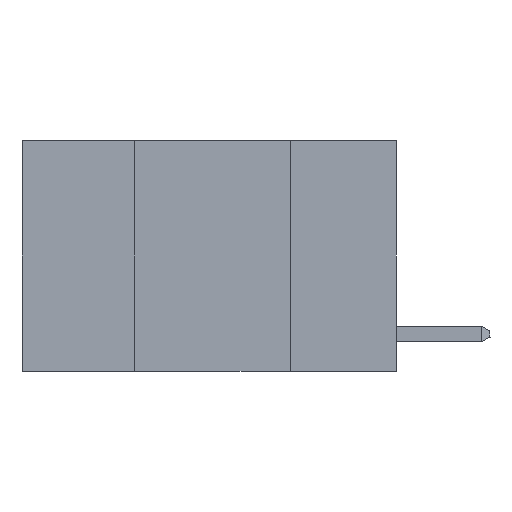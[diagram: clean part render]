
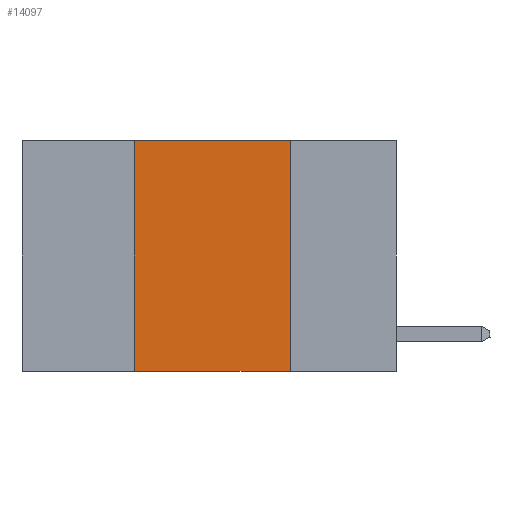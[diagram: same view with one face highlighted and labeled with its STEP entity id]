
A CAD part, left-side view. The second image highlights one B-rep face of the part: STEP entity #14097.
In plain terms, the highlighted planar face has unit normal (-1, 0, 0).
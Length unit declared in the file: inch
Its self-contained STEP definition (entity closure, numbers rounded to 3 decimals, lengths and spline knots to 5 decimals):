
#681 = FACE_OUTER_BOUND ( 'NONE', #6079, .T. ) ;
#1766 = DIRECTION ( 'NONE',  ( 0., -1., 0. ) ) ;
#2060 = ORIENTED_EDGE ( 'NONE', *, *, #2800, .F. ) ;
#2800 = EDGE_CURVE ( 'NONE', #11734, #18228, #6133, .T. ) ;
#3942 = DIRECTION ( 'NONE',  ( 0., 0., -1. ) ) ;
#5501 = DIRECTION ( 'NONE',  ( 0., 0., 1. ) ) ;
#6079 = EDGE_LOOP ( 'NONE', ( #2060, #16665, #7843, #17218 ) ) ;
#6133 = LINE ( 'NONE', #7042, #19045 ) ;
#6497 = LINE ( 'NONE', #8415, #15768 ) ;
#6678 = EDGE_CURVE ( 'NONE', #20570, #18228, #6497, .T. ) ;
#7042 = CARTESIAN_POINT ( 'NONE',  ( 0., 0.17, 0. ) ) ;
#7843 = ORIENTED_EDGE ( 'NONE', *, *, #19462, .F. ) ;
#8415 = CARTESIAN_POINT ( 'NONE',  ( 0., 0.6, -0.37 ) ) ;
#8796 = VECTOR ( 'NONE', #1766, 39.37008 ) ;
#11658 = EDGE_CURVE ( 'NONE', #17234, #11734, #13452, .T. ) ;
#11734 = VERTEX_POINT ( 'NONE', #17817 ) ;
#11872 = DIRECTION ( 'NONE',  ( 0., -1., 0. ) ) ;
#12657 = CARTESIAN_POINT ( 'NONE',  ( 0., 0.6, 0. ) ) ;
#13268 = CARTESIAN_POINT ( 'NONE',  ( 0., 0.42, 0. ) ) ;
#13452 = LINE ( 'NONE', #15804, #8796 ) ;
#14097 = ADVANCED_FACE ( 'NONE', ( #681 ), #19725, .F. ) ;
#14164 = CARTESIAN_POINT ( 'NONE',  ( 0., 0.42, 0. ) ) ;
#14411 = DIRECTION ( 'NONE',  ( 1., 0., 0. ) ) ;
#15167 = CARTESIAN_POINT ( 'NONE',  ( 0., 0.42, -0.37 ) ) ;
#15768 = VECTOR ( 'NONE', #11872, 39.37008 ) ;
#15804 = CARTESIAN_POINT ( 'NONE',  ( 0., 0.6, 0. ) ) ;
#16048 = AXIS2_PLACEMENT_3D ( 'NONE', #12657, #14411, #3942 ) ;
#16252 = CARTESIAN_POINT ( 'NONE',  ( 0., 0.17, -0.37 ) ) ;
#16665 = ORIENTED_EDGE ( 'NONE', *, *, #11658, .F. ) ;
#17218 = ORIENTED_EDGE ( 'NONE', *, *, #6678, .T. ) ;
#17234 = VERTEX_POINT ( 'NONE', #13268 ) ;
#17817 = CARTESIAN_POINT ( 'NONE',  ( 0., 0.17, 0. ) ) ;
#18228 = VERTEX_POINT ( 'NONE', #16252 ) ;
#19045 = VECTOR ( 'NONE', #21062, 39.37008 ) ;
#19462 = EDGE_CURVE ( 'NONE', #20570, #17234, #22184, .T. ) ;
#19725 = PLANE ( 'NONE',  #16048 ) ;
#20570 = VERTEX_POINT ( 'NONE', #15167 ) ;
#21062 = DIRECTION ( 'NONE',  ( 0., 0., -1. ) ) ;
#21111 = VECTOR ( 'NONE', #5501, 39.37008 ) ;
#22184 = LINE ( 'NONE', #14164, #21111 ) ;
